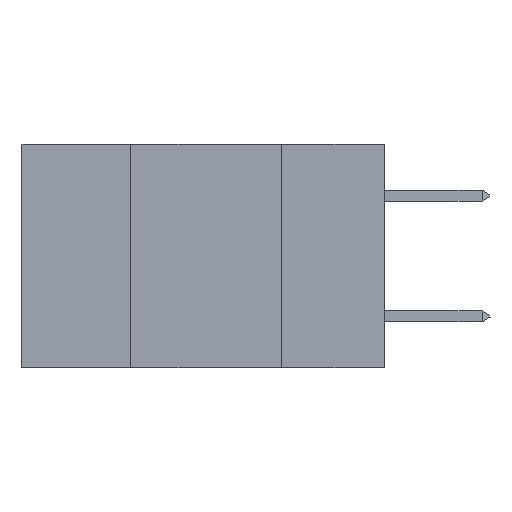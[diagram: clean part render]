
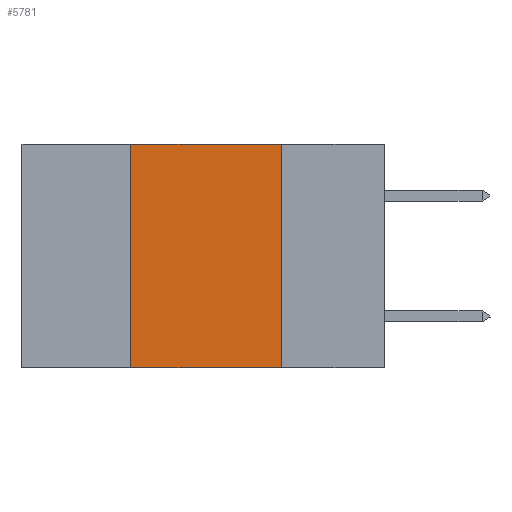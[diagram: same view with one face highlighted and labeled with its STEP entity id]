
A CAD part, left-side view. The second image highlights one B-rep face of the part: STEP entity #5781.
In plain terms, the highlighted planar face has unit normal (-1, 0, 0).
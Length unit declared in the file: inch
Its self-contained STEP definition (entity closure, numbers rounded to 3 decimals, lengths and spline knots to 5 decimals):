
#1152 = DIRECTION ( 'NONE',  ( 0., -1., 0. ) ) ;
#1666 = EDGE_CURVE ( 'NONE', #15979, #27189, #12930, .T. ) ;
#1861 = EDGE_CURVE ( 'NONE', #6224, #16487, #20271, .T. ) ;
#3585 = AXIS2_PLACEMENT_3D ( 'NONE', #22343, #9711, #14056 ) ;
#4602 = CARTESIAN_POINT ( 'NONE',  ( 0., 0.42, -0.37 ) ) ;
#5078 = EDGE_CURVE ( 'NONE', #15979, #6224, #8556, .T. ) ;
#5511 = LINE ( 'NONE', #22523, #12455 ) ;
#5781 = ADVANCED_FACE ( 'NONE', ( #11132 ), #20507, .F. ) ;
#5890 = VECTOR ( 'NONE', #13024, 39.37008 ) ;
#6224 = VERTEX_POINT ( 'NONE', #17668 ) ;
#7481 = ORIENTED_EDGE ( 'NONE', *, *, #5078, .F. ) ;
#8556 = LINE ( 'NONE', #25649, #5890 ) ;
#9711 = DIRECTION ( 'NONE',  ( 1., 0., 0. ) ) ;
#11132 = FACE_OUTER_BOUND ( 'NONE', #21550, .T. ) ;
#11361 = CARTESIAN_POINT ( 'NONE',  ( 0., 0.6, -0.37 ) ) ;
#12085 = DIRECTION ( 'NONE',  ( 0., -1., 0. ) ) ;
#12455 = VECTOR ( 'NONE', #24725, 39.37008 ) ;
#12930 = LINE ( 'NONE', #11361, #17581 ) ;
#13024 = DIRECTION ( 'NONE',  ( 0., 0., 1. ) ) ;
#14056 = DIRECTION ( 'NONE',  ( 0., 0., -1. ) ) ;
#15979 = VERTEX_POINT ( 'NONE', #4602 ) ;
#16487 = VERTEX_POINT ( 'NONE', #20852 ) ;
#16582 = CARTESIAN_POINT ( 'NONE',  ( 0., 0.17, -0.37 ) ) ;
#17581 = VECTOR ( 'NONE', #1152, 39.37008 ) ;
#17668 = CARTESIAN_POINT ( 'NONE',  ( 0., 0.42, 0. ) ) ;
#17801 = ORIENTED_EDGE ( 'NONE', *, *, #1861, .F. ) ;
#20271 = LINE ( 'NONE', #22600, #23554 ) ;
#20507 = PLANE ( 'NONE',  #3585 ) ;
#20852 = CARTESIAN_POINT ( 'NONE',  ( 0., 0.17, 0. ) ) ;
#21550 = EDGE_LOOP ( 'NONE', ( #26414, #17801, #7481, #25281 ) ) ;
#22343 = CARTESIAN_POINT ( 'NONE',  ( 0., 0.6, 0. ) ) ;
#22523 = CARTESIAN_POINT ( 'NONE',  ( 0., 0.17, 0. ) ) ;
#22600 = CARTESIAN_POINT ( 'NONE',  ( 0., 0.6, 0. ) ) ;
#23479 = EDGE_CURVE ( 'NONE', #16487, #27189, #5511, .T. ) ;
#23554 = VECTOR ( 'NONE', #12085, 39.37008 ) ;
#24725 = DIRECTION ( 'NONE',  ( 0., 0., -1. ) ) ;
#25281 = ORIENTED_EDGE ( 'NONE', *, *, #1666, .T. ) ;
#25649 = CARTESIAN_POINT ( 'NONE',  ( 0., 0.42, 0. ) ) ;
#26414 = ORIENTED_EDGE ( 'NONE', *, *, #23479, .F. ) ;
#27189 = VERTEX_POINT ( 'NONE', #16582 ) ;
